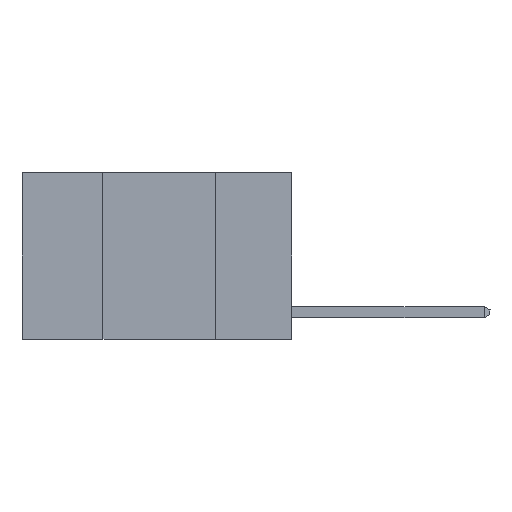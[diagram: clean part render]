
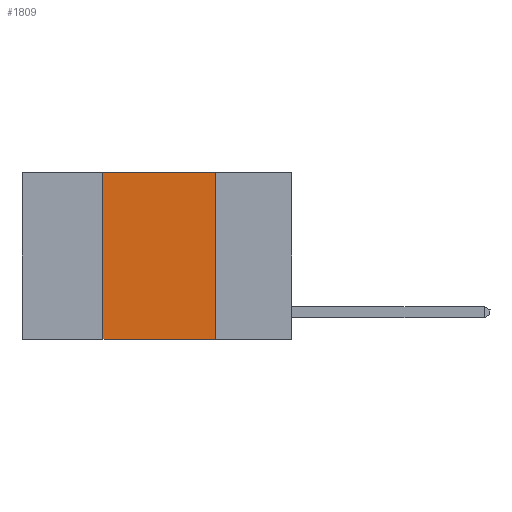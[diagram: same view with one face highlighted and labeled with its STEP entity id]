
A CAD part, left-side view. The second image highlights one B-rep face of the part: STEP entity #1809.
In plain terms, the highlighted planar face has unit normal (-1, 0, 0).
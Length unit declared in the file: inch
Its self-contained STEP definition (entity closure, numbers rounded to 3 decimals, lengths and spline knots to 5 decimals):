
#112 = LINE ( 'NONE', #7483, #3618 ) ;
#467 = LINE ( 'NONE', #595, #944 ) ;
#595 = CARTESIAN_POINT ( 'NONE',  ( 0., 0.6, 0. ) ) ;
#605 = ORIENTED_EDGE ( 'NONE', *, *, #4185, .F. ) ;
#679 = VERTEX_POINT ( 'NONE', #4732 ) ;
#944 = VECTOR ( 'NONE', #6892, 39.37008 ) ;
#1231 = DIRECTION ( 'NONE',  ( 0., 0., 1. ) ) ;
#1809 = ADVANCED_FACE ( 'NONE', ( #9990 ), #3774, .F. ) ;
#2049 = DIRECTION ( 'NONE',  ( 0., 0., -1. ) ) ;
#2197 = CARTESIAN_POINT ( 'NONE',  ( 0., 0.6, -0.37 ) ) ;
#2416 = VECTOR ( 'NONE', #2049, 39.37008 ) ;
#2966 = AXIS2_PLACEMENT_3D ( 'NONE', #6086, #4546, #3712 ) ;
#3266 = VERTEX_POINT ( 'NONE', #5996 ) ;
#3618 = VECTOR ( 'NONE', #1231, 39.37008 ) ;
#3712 = DIRECTION ( 'NONE',  ( 0., 0., -1. ) ) ;
#3774 = PLANE ( 'NONE',  #2966 ) ;
#4185 = EDGE_CURVE ( 'NONE', #679, #7167, #467, .T. ) ;
#4411 = ORIENTED_EDGE ( 'NONE', *, *, #7611, .F. ) ;
#4454 = CARTESIAN_POINT ( 'NONE',  ( 0., 0.42, -0.37 ) ) ;
#4546 = DIRECTION ( 'NONE',  ( 1., 0., 0. ) ) ;
#4732 = CARTESIAN_POINT ( 'NONE',  ( 0., 0.42, 0. ) ) ;
#5278 = CARTESIAN_POINT ( 'NONE',  ( 0., 0.17, 0. ) ) ;
#5354 = EDGE_LOOP ( 'NONE', ( #5600, #605, #4411, #9427 ) ) ;
#5600 = ORIENTED_EDGE ( 'NONE', *, *, #7722, .F. ) ;
#5872 = DIRECTION ( 'NONE',  ( 0., -1., 0. ) ) ;
#5996 = CARTESIAN_POINT ( 'NONE',  ( 0., 0.17, -0.37 ) ) ;
#6086 = CARTESIAN_POINT ( 'NONE',  ( 0., 0.6, 0. ) ) ;
#6892 = DIRECTION ( 'NONE',  ( 0., -1., 0. ) ) ;
#7153 = VECTOR ( 'NONE', #5872, 39.37008 ) ;
#7167 = VERTEX_POINT ( 'NONE', #5278 ) ;
#7199 = LINE ( 'NONE', #8357, #2416 ) ;
#7483 = CARTESIAN_POINT ( 'NONE',  ( 0., 0.42, 0. ) ) ;
#7611 = EDGE_CURVE ( 'NONE', #10122, #679, #112, .T. ) ;
#7722 = EDGE_CURVE ( 'NONE', #7167, #3266, #7199, .T. ) ;
#8357 = CARTESIAN_POINT ( 'NONE',  ( 0., 0.17, 0. ) ) ;
#9427 = ORIENTED_EDGE ( 'NONE', *, *, #10015, .T. ) ;
#9513 = LINE ( 'NONE', #2197, #7153 ) ;
#9990 = FACE_OUTER_BOUND ( 'NONE', #5354, .T. ) ;
#10015 = EDGE_CURVE ( 'NONE', #10122, #3266, #9513, .T. ) ;
#10122 = VERTEX_POINT ( 'NONE', #4454 ) ;
